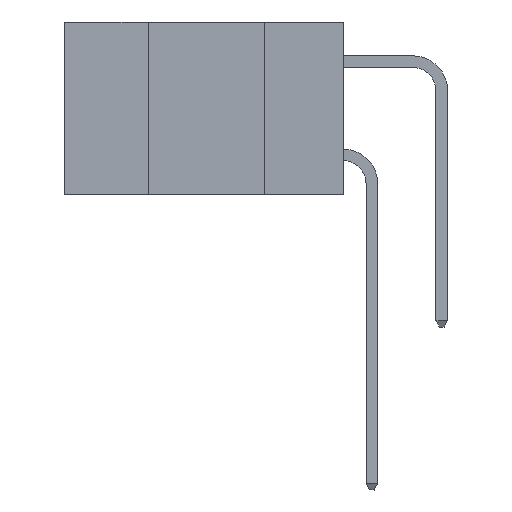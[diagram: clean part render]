
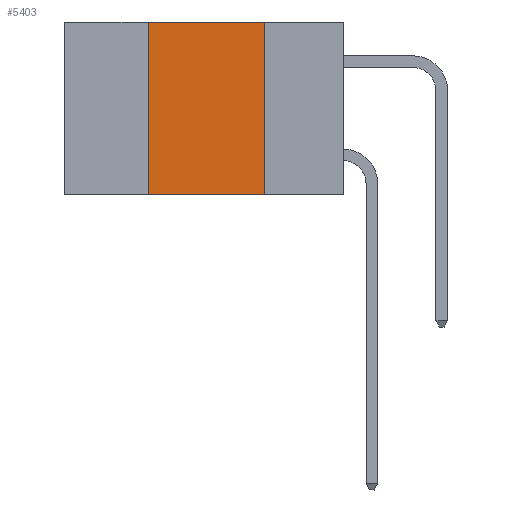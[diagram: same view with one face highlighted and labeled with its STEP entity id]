
A CAD part, left-side view. The second image highlights one B-rep face of the part: STEP entity #5403.
In plain terms, the highlighted planar face has unit normal (-1, 0, 0).
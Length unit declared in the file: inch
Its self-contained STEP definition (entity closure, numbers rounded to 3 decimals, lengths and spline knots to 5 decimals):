
#6 = DIRECTION ( 'NONE',  ( 0., -1., 0. ) ) ;
#719 = CARTESIAN_POINT ( 'NONE',  ( 0., 0.6, -0.37 ) ) ;
#1683 = VECTOR ( 'NONE', #6, 39.37008 ) ;
#2204 = VECTOR ( 'NONE', #17359, 39.37008 ) ;
#2467 = VERTEX_POINT ( 'NONE', #18865 ) ;
#2889 = LINE ( 'NONE', #719, #1683 ) ;
#3070 = CARTESIAN_POINT ( 'NONE',  ( 0., 0.42, -0.37 ) ) ;
#3488 = CARTESIAN_POINT ( 'NONE',  ( 0., 0.42, -0.37 ) ) ;
#5161 = CARTESIAN_POINT ( 'NONE',  ( 0., 0.17, 0. ) ) ;
#5354 = EDGE_CURVE ( 'NONE', #17582, #20517, #2889, .T. ) ;
#5403 = ADVANCED_FACE ( 'NONE', ( #14783 ), #7580, .F. ) ;
#6321 = CARTESIAN_POINT ( 'NONE',  ( 0., 0.17, -0.37 ) ) ;
#7580 = PLANE ( 'NONE',  #16935 ) ;
#8332 = EDGE_CURVE ( 'NONE', #21941, #20517, #12106, .T. ) ;
#8715 = DIRECTION ( 'NONE',  ( 0., 0., 1. ) ) ;
#8974 = ORIENTED_EDGE ( 'NONE', *, *, #16965, .F. ) ;
#9264 = ORIENTED_EDGE ( 'NONE', *, *, #12035, .F. ) ;
#9418 = DIRECTION ( 'NONE',  ( 1., 0., 0. ) ) ;
#11067 = DIRECTION ( 'NONE',  ( 0., -1., 0. ) ) ;
#11580 = VECTOR ( 'NONE', #11067, 39.37008 ) ;
#12035 = EDGE_CURVE ( 'NONE', #17582, #2467, #17888, .T. ) ;
#12106 = LINE ( 'NONE', #6321, #2204 ) ;
#14783 = FACE_OUTER_BOUND ( 'NONE', #14846, .T. ) ;
#14846 = EDGE_LOOP ( 'NONE', ( #18136, #8974, #9264, #16453 ) ) ;
#16453 = ORIENTED_EDGE ( 'NONE', *, *, #5354, .T. ) ;
#16935 = AXIS2_PLACEMENT_3D ( 'NONE', #20381, #9418, #22195 ) ;
#16965 = EDGE_CURVE ( 'NONE', #2467, #21941, #20730, .T. ) ;
#17359 = DIRECTION ( 'NONE',  ( 0., 0., -1. ) ) ;
#17582 = VERTEX_POINT ( 'NONE', #3488 ) ;
#17888 = LINE ( 'NONE', #3070, #18979 ) ;
#18136 = ORIENTED_EDGE ( 'NONE', *, *, #8332, .F. ) ;
#18865 = CARTESIAN_POINT ( 'NONE',  ( 0., 0.42, 0. ) ) ;
#18979 = VECTOR ( 'NONE', #8715, 39.37008 ) ;
#20381 = CARTESIAN_POINT ( 'NONE',  ( 0., 0.6, 0. ) ) ;
#20517 = VERTEX_POINT ( 'NONE', #21995 ) ;
#20730 = LINE ( 'NONE', #23778, #11580 ) ;
#21941 = VERTEX_POINT ( 'NONE', #5161 ) ;
#21995 = CARTESIAN_POINT ( 'NONE',  ( 0., 0.17, -0.37 ) ) ;
#22195 = DIRECTION ( 'NONE',  ( 0., 0., -1. ) ) ;
#23778 = CARTESIAN_POINT ( 'NONE',  ( 0., 0.6, 0. ) ) ;
